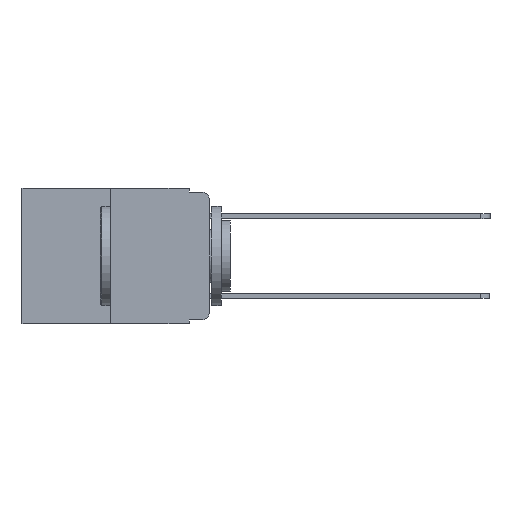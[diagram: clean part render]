
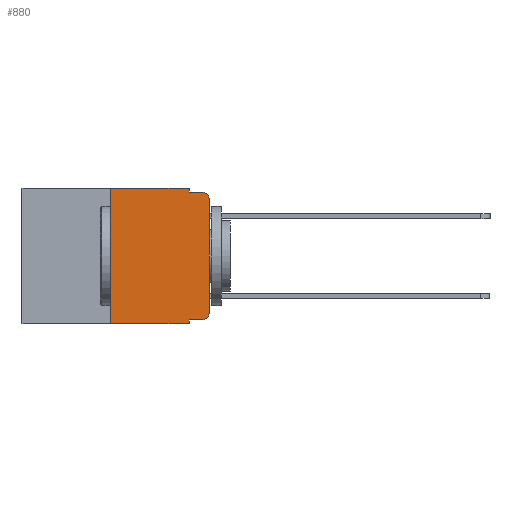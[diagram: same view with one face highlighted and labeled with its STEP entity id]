
A CAD part, left-side view. The second image highlights one B-rep face of the part: STEP entity #880.
In plain terms, the highlighted planar face has unit normal (-1, 0, 0).
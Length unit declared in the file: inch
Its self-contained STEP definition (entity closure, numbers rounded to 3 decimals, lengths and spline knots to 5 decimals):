
#411 = ORIENTED_EDGE ( 'NONE', *, *, #1898, .T. ) ;
#480 = DIRECTION ( 'NONE',  ( 1., 0., 0. ) ) ;
#880 = ADVANCED_FACE ( 'NONE', ( #16129 ), #7246, .F. ) ;
#974 = VERTEX_POINT ( 'NONE', #10218 ) ;
#1022 = EDGE_CURVE ( 'NONE', #14353, #14294, #15111, .T. ) ;
#1400 = EDGE_CURVE ( 'NONE', #5790, #974, #5986, .T. ) ;
#1678 = ORIENTED_EDGE ( 'NONE', *, *, #1874, .T. ) ;
#1755 = EDGE_CURVE ( 'NONE', #15816, #6641, #15277, .T. ) ;
#1776 = EDGE_CURVE ( 'NONE', #6641, #5045, #5063, .T. ) ;
#1821 = EDGE_CURVE ( 'NONE', #11554, #5045, #10327, .T. ) ;
#1839 = EDGE_CURVE ( 'NONE', #14294, #11554, #13674, .T. ) ;
#1848 = EDGE_CURVE ( 'NONE', #5790, #14353, #16269, .T. ) ;
#1871 = EDGE_CURVE ( 'NONE', #16834, #974, #12884, .T. ) ;
#1874 = EDGE_CURVE ( 'NONE', #16834, #16647, #9504, .T. ) ;
#1898 = EDGE_CURVE ( 'NONE', #16647, #15816, #8644, .T. ) ;
#2331 = CARTESIAN_POINT ( 'NONE',  ( 0., 0.051, -0.01 ) ) ;
#3677 = DIRECTION ( 'NONE',  ( 0., -1., 0. ) ) ;
#4464 = CARTESIAN_POINT ( 'NONE',  ( 0., 0.02, -0.313 ) ) ;
#4515 = CARTESIAN_POINT ( 'NONE',  ( 0., 0.051, -0.333 ) ) ;
#4521 = CARTESIAN_POINT ( 'NONE',  ( 0., 0.25, -0.343 ) ) ;
#4589 = ORIENTED_EDGE ( 'NONE', *, *, #1755, .T. ) ;
#5045 = VERTEX_POINT ( 'NONE', #11139 ) ;
#5063 = CIRCLE ( 'NONE', #13676, 0.02 ) ;
#5521 = ORIENTED_EDGE ( 'NONE', *, *, #1776, .T. ) ;
#5731 = VECTOR ( 'NONE', #7014, 39.37008 ) ;
#5790 = VERTEX_POINT ( 'NONE', #4521 ) ;
#5986 = LINE ( 'NONE', #14584, #12704 ) ;
#6218 = DIRECTION ( 'NONE',  ( 0., -1., 0. ) ) ;
#6529 = CARTESIAN_POINT ( 'NONE',  ( 0., 0., -0.03 ) ) ;
#6637 = VECTOR ( 'NONE', #3677, 39.37008 ) ;
#6641 = VERTEX_POINT ( 'NONE', #6529 ) ;
#6692 = AXIS2_PLACEMENT_3D ( 'NONE', #9829, #480, #15189 ) ;
#6861 = DIRECTION ( 'NONE',  ( 0., 0., -1. ) ) ;
#6991 = CARTESIAN_POINT ( 'NONE',  ( 0., 0.25, 0. ) ) ;
#7014 = DIRECTION ( 'NONE',  ( 0., 0., -1. ) ) ;
#7246 = PLANE ( 'NONE',  #6692 ) ;
#7391 = CARTESIAN_POINT ( 'NONE',  ( 0., 0.051, 0. ) ) ;
#7525 = ORIENTED_EDGE ( 'NONE', *, *, #1022, .F. ) ;
#8030 = CARTESIAN_POINT ( 'NONE',  ( 0., 0., 0. ) ) ;
#8142 = AXIS2_PLACEMENT_3D ( 'NONE', #4464, #12856, #13470 ) ;
#8407 = CARTESIAN_POINT ( 'NONE',  ( 0., 0.25, 0. ) ) ;
#8432 = VECTOR ( 'NONE', #12581, 39.37008 ) ;
#8635 = CARTESIAN_POINT ( 'NONE',  ( 0., 0.051, -0.01 ) ) ;
#8644 = CIRCLE ( 'NONE', #8142, 0.02 ) ;
#8692 = CARTESIAN_POINT ( 'NONE',  ( 0., 0.051, 0. ) ) ;
#8748 = DIRECTION ( 'NONE',  ( 0., 0., -1. ) ) ;
#8788 = DIRECTION ( 'NONE',  ( 0., 0., 1. ) ) ;
#9504 = LINE ( 'NONE', #4515, #15860 ) ;
#9727 = CARTESIAN_POINT ( 'NONE',  ( 0., 0.051, 0. ) ) ;
#9829 = CARTESIAN_POINT ( 'NONE',  ( 0., 0.473, 0. ) ) ;
#10218 = CARTESIAN_POINT ( 'NONE',  ( 0., 0.051, -0.343 ) ) ;
#10327 = LINE ( 'NONE', #8635, #6637 ) ;
#10476 = CARTESIAN_POINT ( 'NONE',  ( 0., 0., -0.313 ) ) ;
#10982 = CARTESIAN_POINT ( 'NONE',  ( 0., 0.02, -0.03 ) ) ;
#10996 = DIRECTION ( 'NONE',  ( -1., 0., 0. ) ) ;
#11139 = CARTESIAN_POINT ( 'NONE',  ( 0., 0.02, -0.01 ) ) ;
#11554 = VERTEX_POINT ( 'NONE', #2331 ) ;
#11750 = VECTOR ( 'NONE', #6218, 39.37008 ) ;
#11784 = DIRECTION ( 'NONE',  ( 0., -1., 0. ) ) ;
#12581 = DIRECTION ( 'NONE',  ( 0., 0., 1. ) ) ;
#12704 = VECTOR ( 'NONE', #11784, 39.37008 ) ;
#12856 = DIRECTION ( 'NONE',  ( -1., 0., 0. ) ) ;
#12884 = LINE ( 'NONE', #7391, #5731 ) ;
#13278 = VECTOR ( 'NONE', #8748, 39.37008 ) ;
#13380 = ORIENTED_EDGE ( 'NONE', *, *, #1871, .F. ) ;
#13470 = DIRECTION ( 'NONE',  ( 0., 0., -1. ) ) ;
#13674 = LINE ( 'NONE', #8692, #13278 ) ;
#13676 = AXIS2_PLACEMENT_3D ( 'NONE', #10982, #10996, #6861 ) ;
#14052 = ORIENTED_EDGE ( 'NONE', *, *, #1839, .F. ) ;
#14274 = CARTESIAN_POINT ( 'NONE',  ( 0., 0.051, -0.333 ) ) ;
#14294 = VERTEX_POINT ( 'NONE', #9727 ) ;
#14353 = VERTEX_POINT ( 'NONE', #8407 ) ;
#14496 = ORIENTED_EDGE ( 'NONE', *, *, #1400, .T. ) ;
#14584 = CARTESIAN_POINT ( 'NONE',  ( 0., 0.473, -0.343 ) ) ;
#15111 = LINE ( 'NONE', #15192, #11750 ) ;
#15189 = DIRECTION ( 'NONE',  ( 0., 0., -1. ) ) ;
#15192 = CARTESIAN_POINT ( 'NONE',  ( 0., 0.473, 0. ) ) ;
#15277 = LINE ( 'NONE', #8030, #8432 ) ;
#15307 = DIRECTION ( 'NONE',  ( 0., -1., 0. ) ) ;
#15337 = CARTESIAN_POINT ( 'NONE',  ( 0., 0.02, -0.333 ) ) ;
#15816 = VERTEX_POINT ( 'NONE', #10476 ) ;
#15860 = VECTOR ( 'NONE', #15307, 39.37008 ) ;
#16129 = FACE_OUTER_BOUND ( 'NONE', #16824, .T. ) ;
#16269 = LINE ( 'NONE', #6991, #16661 ) ;
#16286 = ORIENTED_EDGE ( 'NONE', *, *, #1848, .F. ) ;
#16644 = ORIENTED_EDGE ( 'NONE', *, *, #1821, .F. ) ;
#16647 = VERTEX_POINT ( 'NONE', #15337 ) ;
#16661 = VECTOR ( 'NONE', #8788, 39.37008 ) ;
#16824 = EDGE_LOOP ( 'NONE', ( #4589, #5521, #16644, #14052, #7525, #16286, #14496, #13380, #1678, #411 ) ) ;
#16834 = VERTEX_POINT ( 'NONE', #14274 ) ;
